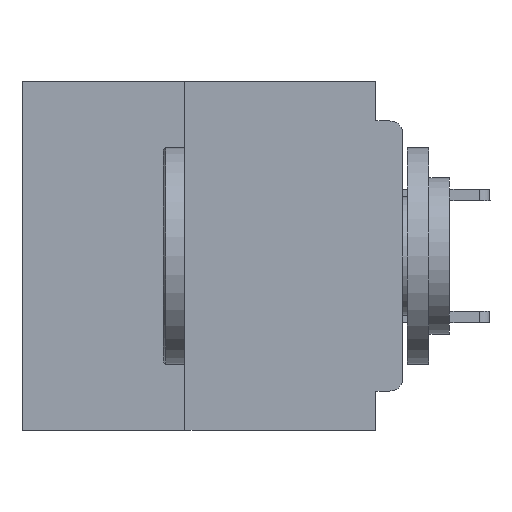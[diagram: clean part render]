
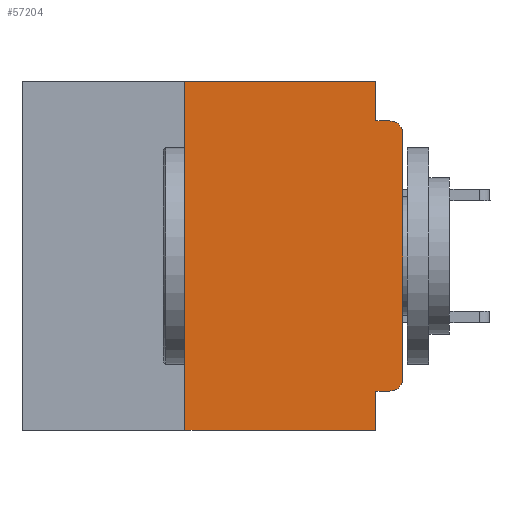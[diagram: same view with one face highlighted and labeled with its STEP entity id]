
A CAD part, left-side view. The second image highlights one B-rep face of the part: STEP entity #57204.
In plain terms, the highlighted planar face has unit normal (-1, 0, 0).
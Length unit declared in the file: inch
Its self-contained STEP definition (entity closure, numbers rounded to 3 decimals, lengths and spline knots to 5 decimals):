
#745 = ORIENTED_EDGE ( 'NONE', *, *, #48189, .T. ) ;
#864 = CARTESIAN_POINT ( 'NONE',  ( 0., 0.015, -0.045 ) ) ;
#969 = CARTESIAN_POINT ( 'NONE',  ( 0., 0.031, -0.355 ) ) ;
#1324 = ORIENTED_EDGE ( 'NONE', *, *, #40049, .F. ) ;
#1440 = LINE ( 'NONE', #38586, #26984 ) ;
#3144 = CARTESIAN_POINT ( 'NONE',  ( 0., 0.437, 0. ) ) ;
#3224 = DIRECTION ( 'NONE',  ( 0., -1., 0. ) ) ;
#3513 = CARTESIAN_POINT ( 'NONE',  ( 0., 0.015, -0.06 ) ) ;
#4165 = EDGE_CURVE ( 'NONE', #36793, #17871, #36822, .T. ) ;
#5033 = VECTOR ( 'NONE', #41887, 39.37008 ) ;
#5552 = CIRCLE ( 'NONE', #14289, 0.015 ) ;
#6264 = VECTOR ( 'NONE', #3224, 39.37008 ) ;
#7242 = VERTEX_POINT ( 'NONE', #969 ) ;
#8356 = DIRECTION ( 'NONE',  ( 0., 0., -1. ) ) ;
#8739 = DIRECTION ( 'NONE',  ( 0., 0., -1. ) ) ;
#9185 = DIRECTION ( 'NONE',  ( 0., 0., 1. ) ) ;
#9655 = DIRECTION ( 'NONE',  ( 0., 1., 0. ) ) ;
#10071 = CARTESIAN_POINT ( 'NONE',  ( 0., 0.25, 0. ) ) ;
#11161 = CARTESIAN_POINT ( 'NONE',  ( 0., 0., 0. ) ) ;
#11162 = EDGE_CURVE ( 'NONE', #7242, #16596, #37361, .T. ) ;
#11597 = ORIENTED_EDGE ( 'NONE', *, *, #11162, .F. ) ;
#13285 = PLANE ( 'NONE',  #21963 ) ;
#14289 = AXIS2_PLACEMENT_3D ( 'NONE', #3513, #39176, #8739 ) ;
#14454 = VERTEX_POINT ( 'NONE', #10071 ) ;
#14724 = CARTESIAN_POINT ( 'NONE',  ( 0., 0.437, 0. ) ) ;
#14961 = VECTOR ( 'NONE', #9655, 39.37008 ) ;
#16056 = CARTESIAN_POINT ( 'NONE',  ( 0., 0.25, -0.4 ) ) ;
#16202 = DIRECTION ( 'NONE',  ( -1., 0., 0. ) ) ;
#16596 = VERTEX_POINT ( 'NONE', #62904 ) ;
#17871 = VERTEX_POINT ( 'NONE', #52779 ) ;
#18706 = LINE ( 'NONE', #36797, #5033 ) ;
#19159 = DIRECTION ( 'NONE',  ( 0., 0., -1. ) ) ;
#19902 = LINE ( 'NONE', #44014, #6264 ) ;
#20986 = ORIENTED_EDGE ( 'NONE', *, *, #37745, .T. ) ;
#21186 = CARTESIAN_POINT ( 'NONE',  ( 0., 0.031, 0. ) ) ;
#21422 = EDGE_CURVE ( 'NONE', #30812, #14454, #18706, .T. ) ;
#21743 = ORIENTED_EDGE ( 'NONE', *, *, #21422, .F. ) ;
#21963 = AXIS2_PLACEMENT_3D ( 'NONE', #3144, #38809, #8356 ) ;
#22049 = EDGE_LOOP ( 'NONE', ( #48894, #42455, #1324, #52451, #52067, #21743, #20986, #11597, #26045, #745 ) ) ;
#22259 = VECTOR ( 'NONE', #19159, 39.37008 ) ;
#23117 = LINE ( 'NONE', #14724, #48566 ) ;
#23328 = VECTOR ( 'NONE', #9185, 39.37008 ) ;
#24376 = LINE ( 'NONE', #28050, #63294 ) ;
#24977 = CARTESIAN_POINT ( 'NONE',  ( 0., 0.015, -0.355 ) ) ;
#26045 = ORIENTED_EDGE ( 'NONE', *, *, #64136, .F. ) ;
#26274 = CIRCLE ( 'NONE', #46682, 0.015 ) ;
#26984 = VECTOR ( 'NONE', #43705, 39.37008 ) ;
#28050 = CARTESIAN_POINT ( 'NONE',  ( 0., 0.031, 0. ) ) ;
#30627 = EDGE_CURVE ( 'NONE', #14454, #51194, #23117, .T. ) ;
#30812 = VERTEX_POINT ( 'NONE', #16056 ) ;
#33203 = DIRECTION ( 'NONE',  ( 0., 0., -1. ) ) ;
#33964 = EDGE_CURVE ( 'NONE', #51194, #47214, #24376, .T. ) ;
#36793 = VERTEX_POINT ( 'NONE', #51155 ) ;
#36797 = CARTESIAN_POINT ( 'NONE',  ( 0., 0.25, -0.4 ) ) ;
#36822 = LINE ( 'NONE', #11161, #23328 ) ;
#37361 = LINE ( 'NONE', #59769, #22259 ) ;
#37745 = EDGE_CURVE ( 'NONE', #30812, #16596, #1440, .T. ) ;
#38586 = CARTESIAN_POINT ( 'NONE',  ( 0., 0.437, -0.4 ) ) ;
#38809 = DIRECTION ( 'NONE',  ( 1., 0., 0. ) ) ;
#39176 = DIRECTION ( 'NONE',  ( -1., 0., 0. ) ) ;
#39418 = EDGE_CURVE ( 'NONE', #17871, #45283, #5552, .T. ) ;
#40049 = EDGE_CURVE ( 'NONE', #47214, #45283, #19902, .T. ) ;
#40076 = CARTESIAN_POINT ( 'NONE',  ( 0., 0., -0.355 ) ) ;
#41370 = CARTESIAN_POINT ( 'NONE',  ( 0., 0.031, -0.045 ) ) ;
#41887 = DIRECTION ( 'NONE',  ( 0., 0., 1. ) ) ;
#41980 = LINE ( 'NONE', #40076, #14961 ) ;
#42455 = ORIENTED_EDGE ( 'NONE', *, *, #39418, .T. ) ;
#43705 = DIRECTION ( 'NONE',  ( 0., -1., 0. ) ) ;
#44014 = CARTESIAN_POINT ( 'NONE',  ( 0., 0., -0.045 ) ) ;
#45283 = VERTEX_POINT ( 'NONE', #864 ) ;
#46640 = CARTESIAN_POINT ( 'NONE',  ( 0., 0.015, -0.34 ) ) ;
#46682 = AXIS2_PLACEMENT_3D ( 'NONE', #46640, #16202, #51688 ) ;
#47074 = VERTEX_POINT ( 'NONE', #24977 ) ;
#47214 = VERTEX_POINT ( 'NONE', #41370 ) ;
#48189 = EDGE_CURVE ( 'NONE', #47074, #36793, #26274, .T. ) ;
#48566 = VECTOR ( 'NONE', #65532, 39.37008 ) ;
#48894 = ORIENTED_EDGE ( 'NONE', *, *, #4165, .T. ) ;
#51155 = CARTESIAN_POINT ( 'NONE',  ( 0., 0., -0.34 ) ) ;
#51194 = VERTEX_POINT ( 'NONE', #21186 ) ;
#51688 = DIRECTION ( 'NONE',  ( 0., 0., -1. ) ) ;
#52067 = ORIENTED_EDGE ( 'NONE', *, *, #30627, .F. ) ;
#52451 = ORIENTED_EDGE ( 'NONE', *, *, #33964, .F. ) ;
#52779 = CARTESIAN_POINT ( 'NONE',  ( 0., 0., -0.06 ) ) ;
#57204 = ADVANCED_FACE ( 'NONE', ( #64345 ), #13285, .F. ) ;
#59769 = CARTESIAN_POINT ( 'NONE',  ( 0., 0.031, -0.4 ) ) ;
#62904 = CARTESIAN_POINT ( 'NONE',  ( 0., 0.031, -0.4 ) ) ;
#63294 = VECTOR ( 'NONE', #33203, 39.37008 ) ;
#64136 = EDGE_CURVE ( 'NONE', #47074, #7242, #41980, .T. ) ;
#64345 = FACE_OUTER_BOUND ( 'NONE', #22049, .T. ) ;
#65532 = DIRECTION ( 'NONE',  ( 0., -1., 0. ) ) ;
